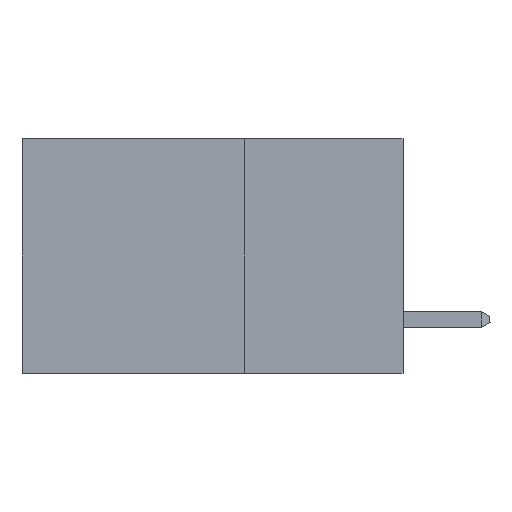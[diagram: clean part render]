
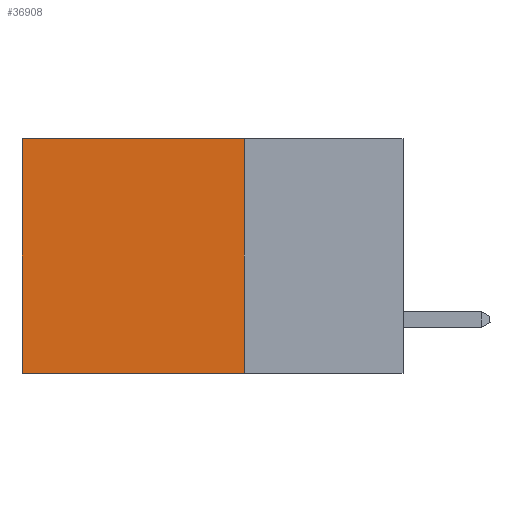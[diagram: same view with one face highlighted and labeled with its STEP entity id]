
A CAD part, left-side view. The second image highlights one B-rep face of the part: STEP entity #36908.
In plain terms, the highlighted planar face has unit normal (-1, 0, 0).
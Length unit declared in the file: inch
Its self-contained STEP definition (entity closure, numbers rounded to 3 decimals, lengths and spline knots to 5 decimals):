
#849 = CARTESIAN_POINT ( 'NONE',  ( 0.2875, 0.25, 0. ) ) ;
#1985 = EDGE_CURVE ( 'NONE', #12399, #13567, #38584, .T. ) ;
#3451 = ORIENTED_EDGE ( 'NONE', *, *, #22256, .F. ) ;
#3639 = DIRECTION ( 'NONE',  ( 0., 1., 0. ) ) ;
#4280 = ORIENTED_EDGE ( 'NONE', *, *, #1985, .T. ) ;
#6003 = EDGE_CURVE ( 'NONE', #13567, #41898, #8960, .T. ) ;
#6578 = LINE ( 'NONE', #27839, #9754 ) ;
#7180 = FACE_OUTER_BOUND ( 'NONE', #34356, .T. ) ;
#8960 = LINE ( 'NONE', #30003, #14147 ) ;
#9066 = CARTESIAN_POINT ( 'NONE',  ( 0.2875, 0.25, 0. ) ) ;
#9754 = VECTOR ( 'NONE', #21276, 39.37008 ) ;
#11943 = CARTESIAN_POINT ( 'NONE',  ( 0.2875, 0.6, 0. ) ) ;
#12399 = VERTEX_POINT ( 'NONE', #9066 ) ;
#13567 = VERTEX_POINT ( 'NONE', #11943 ) ;
#13852 = AXIS2_PLACEMENT_3D ( 'NONE', #43187, #29854, #43030 ) ;
#14147 = VECTOR ( 'NONE', #43038, 39.37008 ) ;
#14722 = ORIENTED_EDGE ( 'NONE', *, *, #27825, .F. ) ;
#14877 = VERTEX_POINT ( 'NONE', #31532 ) ;
#19183 = LINE ( 'NONE', #38728, #33288 ) ;
#21276 = DIRECTION ( 'NONE',  ( 0., 1., 0. ) ) ;
#22256 = EDGE_CURVE ( 'NONE', #12399, #14877, #19183, .T. ) ;
#26555 = DIRECTION ( 'NONE',  ( 0., 0., -1. ) ) ;
#27825 = EDGE_CURVE ( 'NONE', #14877, #41898, #6578, .T. ) ;
#27839 = CARTESIAN_POINT ( 'NONE',  ( 0.2875, 0.25, -0.37 ) ) ;
#29148 = VECTOR ( 'NONE', #3639, 39.37008 ) ;
#29319 = CARTESIAN_POINT ( 'NONE',  ( 0.2875, 0.6, -0.37 ) ) ;
#29854 = DIRECTION ( 'NONE',  ( 1., 0., 0. ) ) ;
#29887 = ORIENTED_EDGE ( 'NONE', *, *, #6003, .T. ) ;
#30003 = CARTESIAN_POINT ( 'NONE',  ( 0.2875, 0.6, 0. ) ) ;
#31532 = CARTESIAN_POINT ( 'NONE',  ( 0.2875, 0.25, -0.37 ) ) ;
#33288 = VECTOR ( 'NONE', #26555, 39.37008 ) ;
#34356 = EDGE_LOOP ( 'NONE', ( #29887, #14722, #3451, #4280 ) ) ;
#36908 = ADVANCED_FACE ( 'NONE', ( #7180 ), #42760, .F. ) ;
#38584 = LINE ( 'NONE', #849, #29148 ) ;
#38728 = CARTESIAN_POINT ( 'NONE',  ( 0.2875, 0.25, 0. ) ) ;
#41898 = VERTEX_POINT ( 'NONE', #29319 ) ;
#42760 = PLANE ( 'NONE',  #13852 ) ;
#43030 = DIRECTION ( 'NONE',  ( 0., 0., -1. ) ) ;
#43038 = DIRECTION ( 'NONE',  ( 0., 0., -1. ) ) ;
#43187 = CARTESIAN_POINT ( 'NONE',  ( 0.2875, 0.25, 0. ) ) ;
